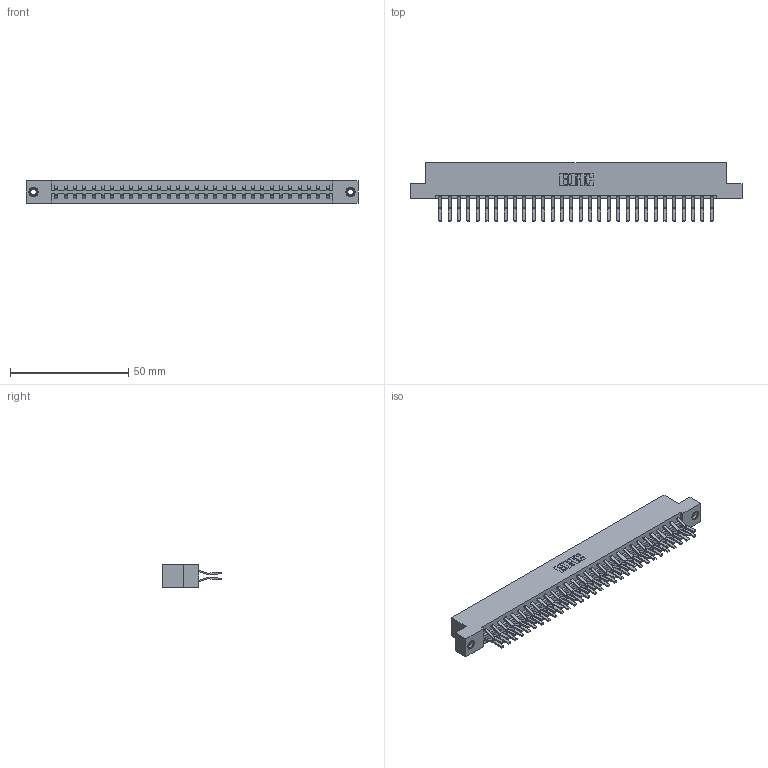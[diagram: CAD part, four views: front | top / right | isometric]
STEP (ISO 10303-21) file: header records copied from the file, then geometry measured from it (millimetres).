
FILE_DESCRIPTION (( 'STEP AP203' ), '1' );
FILE_NAME ('833-060-560-207.STEP', '2020-06-05T04:52:51', ( '' ), ( '' ), 'SwSTEP 2.0', 'SolidWorks 2020', '' );
FILE_SCHEMA (( 'CONFIG_CONTROL_DESIGN' ));
Length unit declared in the file: inch
Products named in the file (4): 833 Part_Flush - .156 Dia - TI; 833-060-560-207; 345-250-001_345-250-005-103; 345-292-001_560 Tail
Assembly tree (63 placements, depth 2):
  833-060-560-207
    833 Part_Flush - .156 Dia - TI
    345-292-001_560 Tail  x60
    345-250-001_345-250-005-103  x2
Bounding box: 140.41 x 24.78 x 9.4 mm (x, y, z)
Volume: 14602.7 mm3; surface area: 18291.1 mm2
Topology: 63 solids, 63 shells, 3414 faces, 10107 edges, 6650 vertices
Faces by surface type: plane 2262, cylinder 1136, cone 12, torus 4
Entity records: 22126 total; most frequent: CARTESIAN_POINT 3665, ORIENTED_EDGE 3594, DIRECTION 3187, EDGE_CURVE 1797, LINE 1645, VECTOR 1645, VERTEX_POINT 1192, AXIS2_PLACEMENT_3D 771
